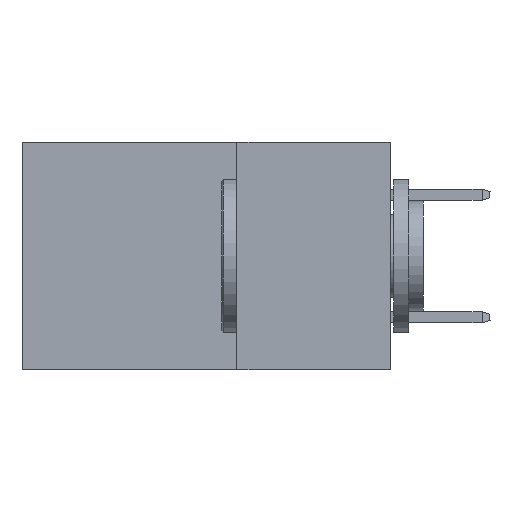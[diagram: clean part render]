
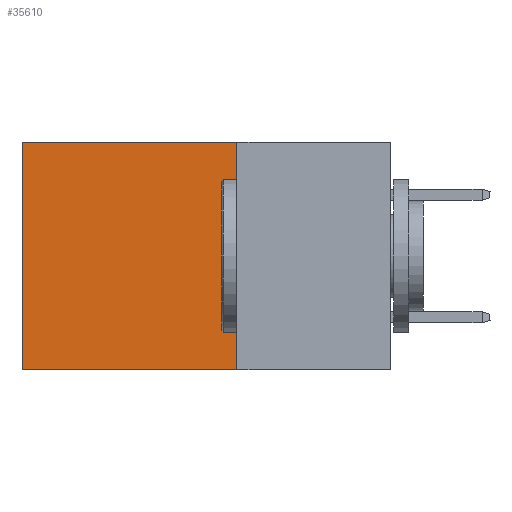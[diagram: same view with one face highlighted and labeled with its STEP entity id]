
A CAD part, left-side view. The second image highlights one B-rep face of the part: STEP entity #35610.
In plain terms, the highlighted planar face has unit normal (-1, 0, 0).
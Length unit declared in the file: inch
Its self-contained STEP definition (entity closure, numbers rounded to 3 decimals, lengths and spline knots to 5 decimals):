
#1694 = CARTESIAN_POINT ( 'NONE',  ( 0.2875, 0.25, 0. ) ) ;
#3869 = ORIENTED_EDGE ( 'NONE', *, *, #8307, .F. ) ;
#3998 = VECTOR ( 'NONE', #23564, 39.37008 ) ;
#5380 = CARTESIAN_POINT ( 'NONE',  ( 0.2875, 0.6, 0. ) ) ;
#5417 = EDGE_CURVE ( 'NONE', #28797, #8372, #28041, .T. ) ;
#6784 = LINE ( 'NONE', #32380, #3998 ) ;
#8144 = AXIS2_PLACEMENT_3D ( 'NONE', #23072, #11319, #14270 ) ;
#8307 = EDGE_CURVE ( 'NONE', #37295, #28797, #37080, .T. ) ;
#8372 = VERTEX_POINT ( 'NONE', #29718 ) ;
#11319 = DIRECTION ( 'NONE',  ( 1., 0., 0. ) ) ;
#11664 = VECTOR ( 'NONE', #31010, 39.37008 ) ;
#12963 = DIRECTION ( 'NONE',  ( 0., 1., 0. ) ) ;
#13666 = ORIENTED_EDGE ( 'NONE', *, *, #5417, .F. ) ;
#14270 = DIRECTION ( 'NONE',  ( 0., 0., -1. ) ) ;
#15495 = VERTEX_POINT ( 'NONE', #5380 ) ;
#17988 = EDGE_LOOP ( 'NONE', ( #23749, #13666, #3869, #21147 ) ) ;
#19288 = CARTESIAN_POINT ( 'NONE',  ( 0.2875, 0.25, -0.37 ) ) ;
#19292 = CARTESIAN_POINT ( 'NONE',  ( 0.2875, 0.25, -0.37 ) ) ;
#21106 = EDGE_CURVE ( 'NONE', #15495, #8372, #6784, .T. ) ;
#21147 = ORIENTED_EDGE ( 'NONE', *, *, #36503, .T. ) ;
#23072 = CARTESIAN_POINT ( 'NONE',  ( 0.2875, 0.25, 0. ) ) ;
#23365 = DIRECTION ( 'NONE',  ( 0., 0., -1. ) ) ;
#23564 = DIRECTION ( 'NONE',  ( 0., 0., -1. ) ) ;
#23749 = ORIENTED_EDGE ( 'NONE', *, *, #21106, .T. ) ;
#28041 = LINE ( 'NONE', #19292, #28536 ) ;
#28532 = CARTESIAN_POINT ( 'NONE',  ( 0.2875, 0.25, 0. ) ) ;
#28536 = VECTOR ( 'NONE', #12963, 39.37008 ) ;
#28568 = CARTESIAN_POINT ( 'NONE',  ( 0.2875, 0.25, 0. ) ) ;
#28797 = VERTEX_POINT ( 'NONE', #19288 ) ;
#29718 = CARTESIAN_POINT ( 'NONE',  ( 0.2875, 0.6, -0.37 ) ) ;
#30169 = VECTOR ( 'NONE', #23365, 39.37008 ) ;
#31010 = DIRECTION ( 'NONE',  ( 0., 1., 0. ) ) ;
#31834 = FACE_OUTER_BOUND ( 'NONE', #17988, .T. ) ;
#32380 = CARTESIAN_POINT ( 'NONE',  ( 0.2875, 0.6, 0. ) ) ;
#35610 = ADVANCED_FACE ( 'NONE', ( #31834 ), #37841, .F. ) ;
#36503 = EDGE_CURVE ( 'NONE', #37295, #15495, #36741, .T. ) ;
#36741 = LINE ( 'NONE', #1694, #11664 ) ;
#37080 = LINE ( 'NONE', #28568, #30169 ) ;
#37295 = VERTEX_POINT ( 'NONE', #28532 ) ;
#37841 = PLANE ( 'NONE',  #8144 ) ;
